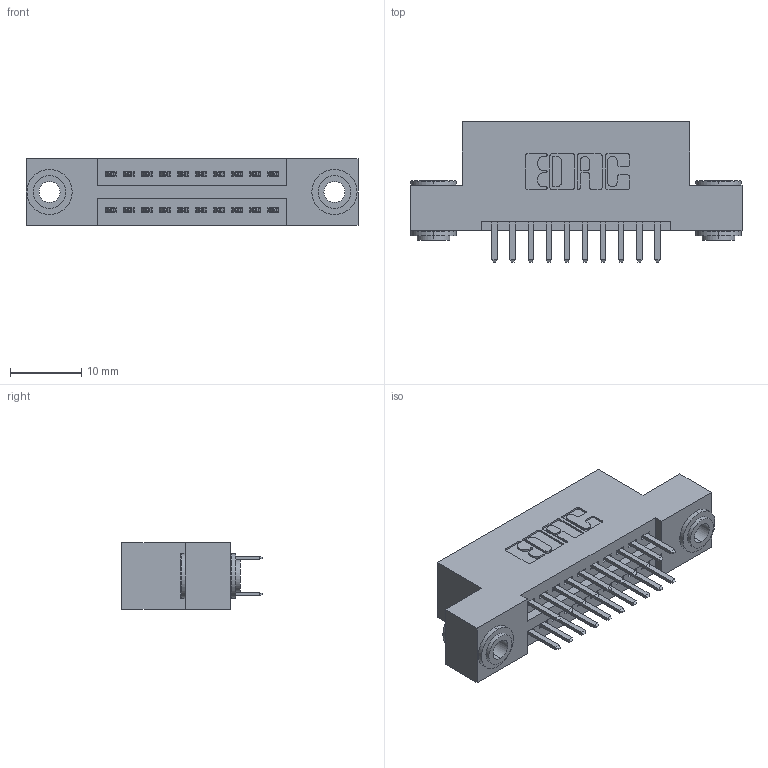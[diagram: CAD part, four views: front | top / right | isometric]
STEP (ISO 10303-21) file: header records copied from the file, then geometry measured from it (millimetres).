
FILE_DESCRIPTION (( 'STEP AP203' ), '1' );
FILE_NAME ('395-020-520-203.STEP', '2018-11-07T14:26:02', ( '' ), ( '' ), 'SwSTEP 2.0', 'SolidWorks 2016', '' );
FILE_SCHEMA (( 'CONFIG_CONTROL_DESIGN' ));
Length unit declared in the file: inch
Products named in the file (4): 345-250-002_345-250-002-102; 345 Part_Flush Mounting Lugs - 0.156 Dia-TH; 395-020-520-203; 345-292-001_345-293-120
Assembly tree (23 placements, depth 2):
  395-020-520-203
    345 Part_Flush Mounting Lugs - 0.156 Dia-TH
    345-292-001_345-293-120  x20
    345-250-002_345-250-002-102  x2
Bounding box: 46.61 x 19.68 x 9.4 mm (x, y, z)
Volume: 4241.2 mm3; surface area: 5835.6 mm2
Topology: 23 solids, 23 shells, 1244 faces, 3557 edges, 2314 vertices
Faces by surface type: plane 790, cylinder 446, cone 8
Entity records: 12918 total; most frequent: CARTESIAN_POINT 2183, ORIENTED_EDGE 2098, DIRECTION 1983, EDGE_CURVE 1049, VECTOR 849, LINE 849, VERTEX_POINT 694, AXIS2_PLACEMENT_3D 567
